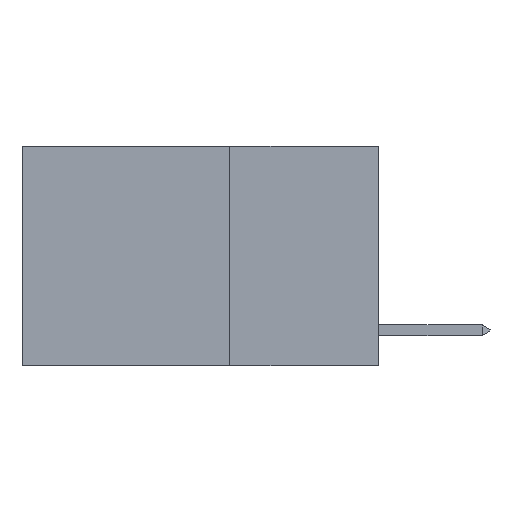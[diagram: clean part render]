
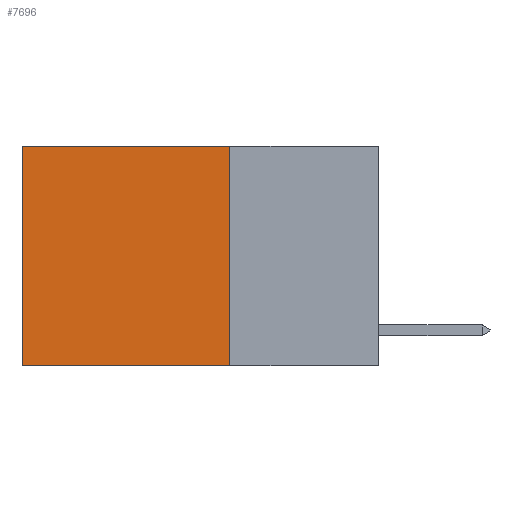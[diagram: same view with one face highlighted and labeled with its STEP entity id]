
A CAD part, left-side view. The second image highlights one B-rep face of the part: STEP entity #7696.
In plain terms, the highlighted planar face has unit normal (-1, 0, 0).
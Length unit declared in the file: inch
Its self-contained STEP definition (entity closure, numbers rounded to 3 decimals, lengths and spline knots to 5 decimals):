
#874 = CARTESIAN_POINT ( 'NONE',  ( 0.2625, 0.6, -0.37 ) ) ;
#1586 = PLANE ( 'NONE',  #17233 ) ;
#1869 = DIRECTION ( 'NONE',  ( 0., 0., -1. ) ) ;
#1988 = EDGE_CURVE ( 'NONE', #4309, #15761, #5308, .T. ) ;
#2263 = ORIENTED_EDGE ( 'NONE', *, *, #5794, .T. ) ;
#2837 = LINE ( 'NONE', #11301, #4414 ) ;
#3360 = VECTOR ( 'NONE', #9811, 39.37008 ) ;
#4079 = CARTESIAN_POINT ( 'NONE',  ( 0.2625, 0.25, -0.37 ) ) ;
#4309 = VERTEX_POINT ( 'NONE', #18313 ) ;
#4414 = VECTOR ( 'NONE', #6872, 39.37008 ) ;
#4566 = EDGE_CURVE ( 'NONE', #6283, #17415, #2837, .T. ) ;
#4700 = VECTOR ( 'NONE', #13699, 39.37008 ) ;
#5308 = LINE ( 'NONE', #11209, #15159 ) ;
#5794 = EDGE_CURVE ( 'NONE', #15761, #17415, #7932, .T. ) ;
#6283 = VERTEX_POINT ( 'NONE', #4079 ) ;
#6872 = DIRECTION ( 'NONE',  ( 0., 1., 0. ) ) ;
#7696 = ADVANCED_FACE ( 'NONE', ( #9127 ), #1586, .F. ) ;
#7932 = LINE ( 'NONE', #16858, #4700 ) ;
#9066 = ORIENTED_EDGE ( 'NONE', *, *, #1988, .T. ) ;
#9127 = FACE_OUTER_BOUND ( 'NONE', #11889, .T. ) ;
#9705 = DIRECTION ( 'NONE',  ( 0., 1., 0. ) ) ;
#9811 = DIRECTION ( 'NONE',  ( 0., 0., -1. ) ) ;
#10528 = ORIENTED_EDGE ( 'NONE', *, *, #4566, .F. ) ;
#11209 = CARTESIAN_POINT ( 'NONE',  ( 0.2625, 0.25, 0. ) ) ;
#11301 = CARTESIAN_POINT ( 'NONE',  ( 0.2625, 0.25, -0.37 ) ) ;
#11399 = CARTESIAN_POINT ( 'NONE',  ( 0.2625, 0.25, 0. ) ) ;
#11447 = LINE ( 'NONE', #11399, #3360 ) ;
#11889 = EDGE_LOOP ( 'NONE', ( #2263, #10528, #12435, #9066 ) ) ;
#12435 = ORIENTED_EDGE ( 'NONE', *, *, #13617, .F. ) ;
#12784 = CARTESIAN_POINT ( 'NONE',  ( 0.2625, 0.6, 0. ) ) ;
#13617 = EDGE_CURVE ( 'NONE', #4309, #6283, #11447, .T. ) ;
#13699 = DIRECTION ( 'NONE',  ( 0., 0., -1. ) ) ;
#14914 = CARTESIAN_POINT ( 'NONE',  ( 0.2625, 0.25, 0. ) ) ;
#15159 = VECTOR ( 'NONE', #9705, 39.37008 ) ;
#15761 = VERTEX_POINT ( 'NONE', #12784 ) ;
#16858 = CARTESIAN_POINT ( 'NONE',  ( 0.2625, 0.6, 0. ) ) ;
#17233 = AXIS2_PLACEMENT_3D ( 'NONE', #14914, #17498, #1869 ) ;
#17415 = VERTEX_POINT ( 'NONE', #874 ) ;
#17498 = DIRECTION ( 'NONE',  ( 1., 0., 0. ) ) ;
#18313 = CARTESIAN_POINT ( 'NONE',  ( 0.2625, 0.25, 0. ) ) ;
